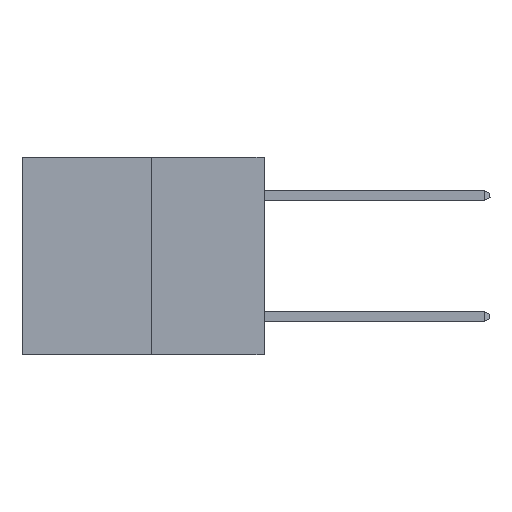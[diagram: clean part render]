
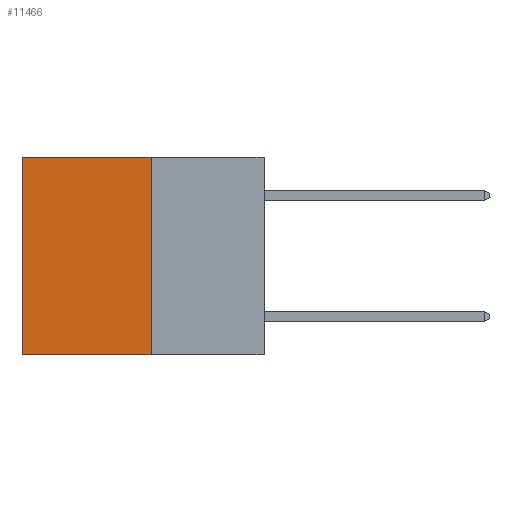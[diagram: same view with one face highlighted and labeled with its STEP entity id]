
A CAD part, left-side view. The second image highlights one B-rep face of the part: STEP entity #11466.
In plain terms, the highlighted planar face has unit normal (-1, 0, 0).
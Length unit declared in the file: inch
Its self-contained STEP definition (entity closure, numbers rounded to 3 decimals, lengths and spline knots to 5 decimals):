
#584 = FACE_OUTER_BOUND ( 'NONE', #25032, .T. ) ;
#3648 = CARTESIAN_POINT ( 'NONE',  ( 0.3165, 0.6, 0. ) ) ;
#3720 = EDGE_CURVE ( 'NONE', #4166, #16121, #16496, .T. ) ;
#4166 = VERTEX_POINT ( 'NONE', #25076 ) ;
#4249 = ORIENTED_EDGE ( 'NONE', *, *, #22469, .T. ) ;
#4644 = VERTEX_POINT ( 'NONE', #27004 ) ;
#4914 = ORIENTED_EDGE ( 'NONE', *, *, #9706, .F. ) ;
#5711 = DIRECTION ( 'NONE',  ( 0., 1., 0. ) ) ;
#6667 = AXIS2_PLACEMENT_3D ( 'NONE', #15932, #18016, #7126 ) ;
#7126 = DIRECTION ( 'NONE',  ( 0., 0., -1. ) ) ;
#7733 = DIRECTION ( 'NONE',  ( 0., 1., 0. ) ) ;
#8186 = VECTOR ( 'NONE', #16472, 39.37008 ) ;
#9494 = LINE ( 'NONE', #14144, #11249 ) ;
#9706 = EDGE_CURVE ( 'NONE', #10875, #4644, #9494, .T. ) ;
#9981 = LINE ( 'NONE', #18758, #8186 ) ;
#10314 = CARTESIAN_POINT ( 'NONE',  ( 0.3165, 0.28, 0. ) ) ;
#10875 = VERTEX_POINT ( 'NONE', #22871 ) ;
#11249 = VECTOR ( 'NONE', #7733, 39.37008 ) ;
#11466 = ADVANCED_FACE ( 'NONE', ( #584 ), #22717, .F. ) ;
#11935 = DIRECTION ( 'NONE',  ( 0., 0., -1. ) ) ;
#14144 = CARTESIAN_POINT ( 'NONE',  ( 0.3165, 0.28, -0.49 ) ) ;
#15253 = ORIENTED_EDGE ( 'NONE', *, *, #16473, .F. ) ;
#15932 = CARTESIAN_POINT ( 'NONE',  ( 0.3165, 0.28, -0.49 ) ) ;
#16121 = VERTEX_POINT ( 'NONE', #3648 ) ;
#16472 = DIRECTION ( 'NONE',  ( 0., 0., -1. ) ) ;
#16473 = EDGE_CURVE ( 'NONE', #4166, #10875, #9981, .T. ) ;
#16496 = LINE ( 'NONE', #10314, #27399 ) ;
#18016 = DIRECTION ( 'NONE',  ( 1., 0., 0. ) ) ;
#18758 = CARTESIAN_POINT ( 'NONE',  ( 0.3165, 0.28, -0.49 ) ) ;
#18847 = CARTESIAN_POINT ( 'NONE',  ( 0.3165, 0.6, -0.49 ) ) ;
#19588 = ORIENTED_EDGE ( 'NONE', *, *, #3720, .T. ) ;
#22409 = VECTOR ( 'NONE', #11935, 39.37008 ) ;
#22469 = EDGE_CURVE ( 'NONE', #16121, #4644, #28012, .T. ) ;
#22717 = PLANE ( 'NONE',  #6667 ) ;
#22871 = CARTESIAN_POINT ( 'NONE',  ( 0.3165, 0.28, -0.49 ) ) ;
#25032 = EDGE_LOOP ( 'NONE', ( #4249, #4914, #15253, #19588 ) ) ;
#25076 = CARTESIAN_POINT ( 'NONE',  ( 0.3165, 0.28, 0. ) ) ;
#27004 = CARTESIAN_POINT ( 'NONE',  ( 0.3165, 0.6, -0.49 ) ) ;
#27399 = VECTOR ( 'NONE', #5711, 39.37008 ) ;
#28012 = LINE ( 'NONE', #18847, #22409 ) ;
